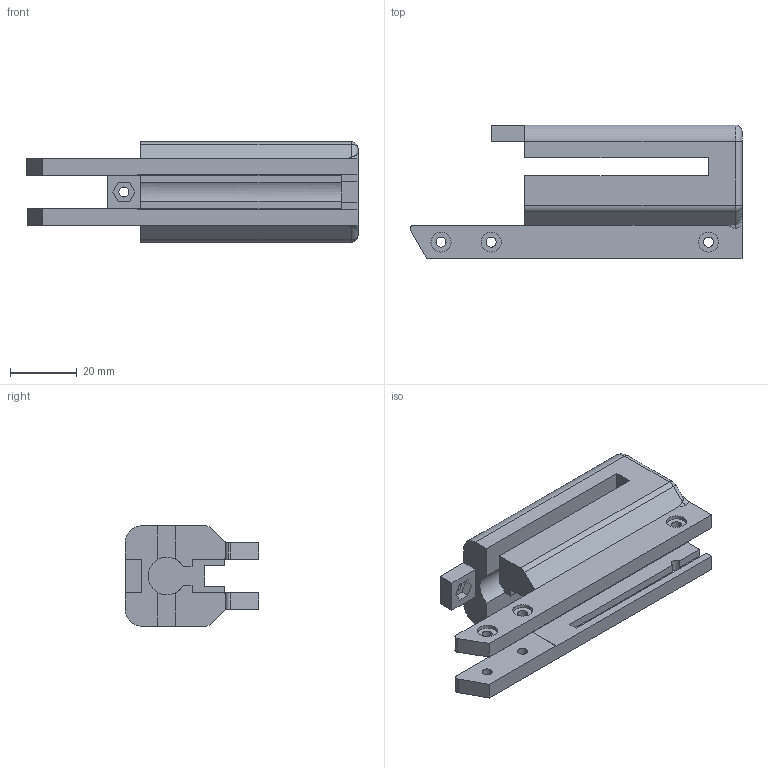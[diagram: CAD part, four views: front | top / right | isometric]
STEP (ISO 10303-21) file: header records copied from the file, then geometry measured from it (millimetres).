
FILE_DESCRIPTION (( 'STEP AP214' ), '1' );
FILE_NAME ('UpperFrame^StikM1.STEP', '2013-09-01T22:36:16', ( 'Asher' ), ( '' ), 'SwSTEP 2.0', 'SolidWorks 2013', '' );
FILE_SCHEMA (( 'AUTOMOTIVE_DESIGN' ));
Length unit declared in the file: millimetre
Products named in the file (1): UpperFrame^StikM1
Bounding box: 99.27 x 40 x 30 mm (x, y, z)
Volume: 46131 mm3; surface area: 18636.7 mm2
Topology: 1 solids, 1 shells, 133 faces, 367 edges, 241 vertices
Faces by surface type: plane 90, cylinder 36, torus 4, bspline 3
Entity records: 4387 total; most frequent: CARTESIAN_POINT 894, ORIENTED_EDGE 734, DIRECTION 699, EDGE_CURVE 367, LINE 275, VECTOR 275, VERTEX_POINT 241, AXIS2_PLACEMENT_3D 212
